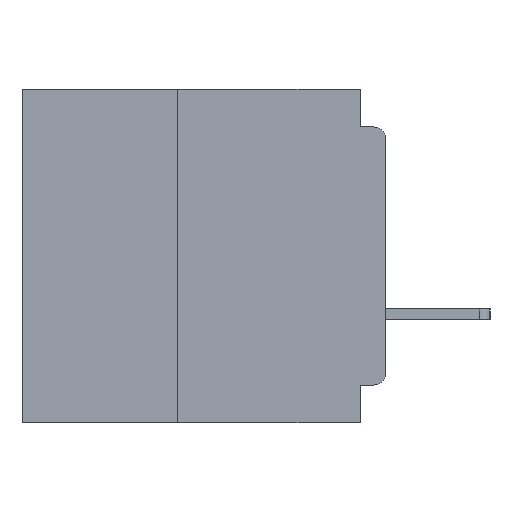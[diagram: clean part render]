
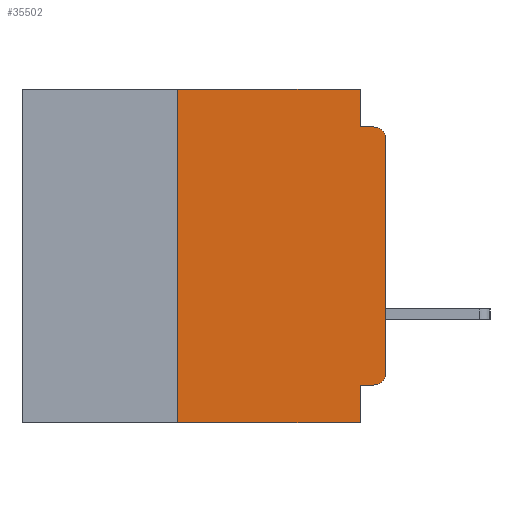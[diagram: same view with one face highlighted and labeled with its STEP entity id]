
A CAD part, left-side view. The second image highlights one B-rep face of the part: STEP entity #35502.
In plain terms, the highlighted planar face has unit normal (-1, 0, 0).
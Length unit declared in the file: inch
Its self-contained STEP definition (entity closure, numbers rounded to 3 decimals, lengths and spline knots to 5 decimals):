
#886 = CARTESIAN_POINT ( 'NONE',  ( 0., 0.031, 0. ) ) ;
#1116 = EDGE_CURVE ( 'NONE', #25299, #67768, #39924, .T. ) ;
#2159 = ORIENTED_EDGE ( 'NONE', *, *, #27250, .F. ) ;
#2162 = LINE ( 'NONE', #23030, #15810 ) ;
#2759 = VERTEX_POINT ( 'NONE', #63885 ) ;
#3203 = ORIENTED_EDGE ( 'NONE', *, *, #26561, .T. ) ;
#3784 = CARTESIAN_POINT ( 'NONE',  ( 0., 0.25, -0.4 ) ) ;
#4816 = CARTESIAN_POINT ( 'NONE',  ( 0., 0.015, -0.34 ) ) ;
#5107 = DIRECTION ( 'NONE',  ( 0., 0., 1. ) ) ;
#7821 = CARTESIAN_POINT ( 'NONE',  ( 0., 0., 0. ) ) ;
#8838 = VECTOR ( 'NONE', #27668, 39.37008 ) ;
#8871 = AXIS2_PLACEMENT_3D ( 'NONE', #62860, #52308, #20349 ) ;
#9958 = VECTOR ( 'NONE', #66413, 39.37008 ) ;
#10243 = DIRECTION ( 'NONE',  ( 0., 0., -1. ) ) ;
#10705 = VERTEX_POINT ( 'NONE', #63209 ) ;
#11110 = CIRCLE ( 'NONE', #56453, 0.015 ) ;
#11983 = ORIENTED_EDGE ( 'NONE', *, *, #35602, .F. ) ;
#12161 = VECTOR ( 'NONE', #50620, 39.37008 ) ;
#15736 = CARTESIAN_POINT ( 'NONE',  ( 0., 0.25, -0.4 ) ) ;
#15810 = VECTOR ( 'NONE', #33794, 39.37008 ) ;
#16350 = DIRECTION ( 'NONE',  ( 0., -1., 0. ) ) ;
#19676 = CARTESIAN_POINT ( 'NONE',  ( 0., 0.25, 0. ) ) ;
#20349 = DIRECTION ( 'NONE',  ( 0., 0., -1. ) ) ;
#21974 = CARTESIAN_POINT ( 'NONE',  ( 0., 0., -0.355 ) ) ;
#22157 = EDGE_LOOP ( 'NONE', ( #50437, #41321, #64095, #32350, #2159, #32194, #69498, #62067, #11983, #3203 ) ) ;
#23030 = CARTESIAN_POINT ( 'NONE',  ( 0., 0.031, -0.4 ) ) ;
#24613 = VERTEX_POINT ( 'NONE', #19676 ) ;
#25299 = VERTEX_POINT ( 'NONE', #3784 ) ;
#25717 = CARTESIAN_POINT ( 'NONE',  ( 0., 0.015, -0.06 ) ) ;
#26392 = DIRECTION ( 'NONE',  ( 0., -1., 0. ) ) ;
#26456 = AXIS2_PLACEMENT_3D ( 'NONE', #4816, #42273, #10243 ) ;
#26561 = EDGE_CURVE ( 'NONE', #43305, #35398, #53160, .T. ) ;
#27250 = EDGE_CURVE ( 'NONE', #24613, #45601, #48894, .T. ) ;
#27643 = LINE ( 'NONE', #15736, #29291 ) ;
#27668 = DIRECTION ( 'NONE',  ( 0., 0., -1. ) ) ;
#28075 = LINE ( 'NONE', #7821, #12161 ) ;
#29291 = VECTOR ( 'NONE', #5107, 39.37008 ) ;
#31093 = DIRECTION ( 'NONE',  ( 0., 0., -1. ) ) ;
#31177 = VECTOR ( 'NONE', #64731, 39.37008 ) ;
#32194 = ORIENTED_EDGE ( 'NONE', *, *, #67797, .F. ) ;
#32350 = ORIENTED_EDGE ( 'NONE', *, *, #58592, .F. ) ;
#32474 = CARTESIAN_POINT ( 'NONE',  ( 0., 0.437, -0.4 ) ) ;
#33616 = VERTEX_POINT ( 'NONE', #58763 ) ;
#33794 = DIRECTION ( 'NONE',  ( 0., 0., -1. ) ) ;
#34710 = VECTOR ( 'NONE', #26392, 39.37008 ) ;
#35398 = VERTEX_POINT ( 'NONE', #40635 ) ;
#35502 = ADVANCED_FACE ( 'NONE', ( #37901 ), #68215, .F. ) ;
#35602 = EDGE_CURVE ( 'NONE', #43305, #33616, #59635, .T. ) ;
#37901 = FACE_OUTER_BOUND ( 'NONE', #22157, .T. ) ;
#38452 = LINE ( 'NONE', #50286, #9958 ) ;
#39007 = LINE ( 'NONE', #886, #8838 ) ;
#39364 = CARTESIAN_POINT ( 'NONE',  ( 0., 0.031, 0. ) ) ;
#39924 = LINE ( 'NONE', #32474, #66679 ) ;
#40635 = CARTESIAN_POINT ( 'NONE',  ( 0., 0., -0.34 ) ) ;
#41321 = ORIENTED_EDGE ( 'NONE', *, *, #51221, .T. ) ;
#42223 = EDGE_CURVE ( 'NONE', #33616, #67768, #2162, .T. ) ;
#42273 = DIRECTION ( 'NONE',  ( -1., 0., 0. ) ) ;
#42326 = CARTESIAN_POINT ( 'NONE',  ( 0., 0.031, -0.4 ) ) ;
#43305 = VERTEX_POINT ( 'NONE', #59131 ) ;
#45039 = EDGE_CURVE ( 'NONE', #35398, #2759, #28075, .T. ) ;
#45601 = VERTEX_POINT ( 'NONE', #39364 ) ;
#48433 = CARTESIAN_POINT ( 'NONE',  ( 0., 0.015, -0.045 ) ) ;
#48894 = LINE ( 'NONE', #63773, #34710 ) ;
#50286 = CARTESIAN_POINT ( 'NONE',  ( 0., 0., -0.045 ) ) ;
#50437 = ORIENTED_EDGE ( 'NONE', *, *, #45039, .T. ) ;
#50620 = DIRECTION ( 'NONE',  ( 0., 0., 1. ) ) ;
#51221 = EDGE_CURVE ( 'NONE', #2759, #60412, #11110, .T. ) ;
#52308 = DIRECTION ( 'NONE',  ( 1., 0., 0. ) ) ;
#53095 = EDGE_CURVE ( 'NONE', #10705, #60412, #38452, .T. ) ;
#53160 = CIRCLE ( 'NONE', #26456, 0.015 ) ;
#56453 = AXIS2_PLACEMENT_3D ( 'NONE', #25717, #63119, #31093 ) ;
#58592 = EDGE_CURVE ( 'NONE', #45601, #10705, #39007, .T. ) ;
#58763 = CARTESIAN_POINT ( 'NONE',  ( 0., 0.031, -0.355 ) ) ;
#59131 = CARTESIAN_POINT ( 'NONE',  ( 0., 0.015, -0.355 ) ) ;
#59635 = LINE ( 'NONE', #21974, #31177 ) ;
#60412 = VERTEX_POINT ( 'NONE', #48433 ) ;
#62067 = ORIENTED_EDGE ( 'NONE', *, *, #42223, .F. ) ;
#62860 = CARTESIAN_POINT ( 'NONE',  ( 0., 0.437, 0. ) ) ;
#63119 = DIRECTION ( 'NONE',  ( -1., 0., 0. ) ) ;
#63209 = CARTESIAN_POINT ( 'NONE',  ( 0., 0.031, -0.045 ) ) ;
#63773 = CARTESIAN_POINT ( 'NONE',  ( 0., 0.437, 0. ) ) ;
#63885 = CARTESIAN_POINT ( 'NONE',  ( 0., 0., -0.06 ) ) ;
#64095 = ORIENTED_EDGE ( 'NONE', *, *, #53095, .F. ) ;
#64731 = DIRECTION ( 'NONE',  ( 0., 1., 0. ) ) ;
#66413 = DIRECTION ( 'NONE',  ( 0., -1., 0. ) ) ;
#66679 = VECTOR ( 'NONE', #16350, 39.37008 ) ;
#67768 = VERTEX_POINT ( 'NONE', #42326 ) ;
#67797 = EDGE_CURVE ( 'NONE', #25299, #24613, #27643, .T. ) ;
#68215 = PLANE ( 'NONE',  #8871 ) ;
#69498 = ORIENTED_EDGE ( 'NONE', *, *, #1116, .T. ) ;
